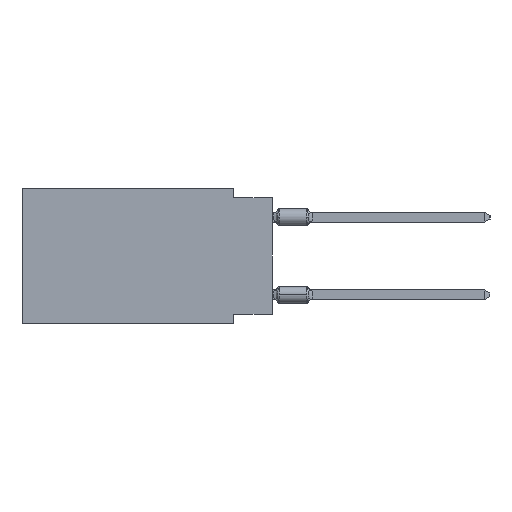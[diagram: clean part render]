
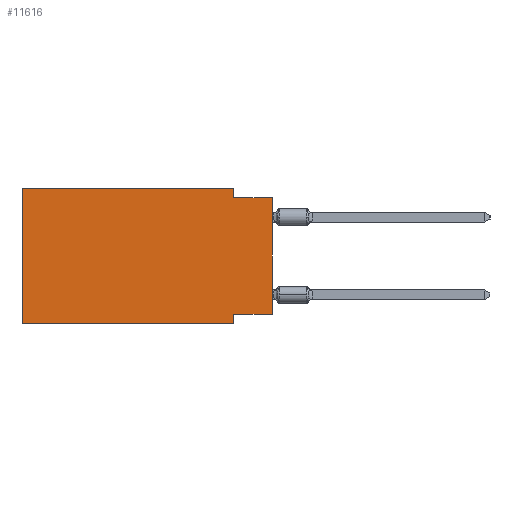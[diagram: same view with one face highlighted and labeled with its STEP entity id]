
A CAD part, left-side view. The second image highlights one B-rep face of the part: STEP entity #11616.
In plain terms, the highlighted planar face has unit normal (-1, 0, 0).
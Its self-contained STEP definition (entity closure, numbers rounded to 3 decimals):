
#1802 = CARTESIAN_POINT ( 'NONE',  ( 0., 0., 0. ) ) ;
#1859 = DIRECTION ( 'NONE',  ( 0., -1., 0. ) ) ;
#2640 = VERTEX_POINT ( 'NONE', #13204 ) ;
#3303 = ORIENTED_EDGE ( 'NONE', *, *, #38712, .F. ) ;
#4623 = VECTOR ( 'NONE', #34540, 1000. ) ;
#5333 = CARTESIAN_POINT ( 'NONE',  ( 0., 2.54, -8.89 ) ) ;
#6080 = VERTEX_POINT ( 'NONE', #53023 ) ;
#6887 = CARTESIAN_POINT ( 'NONE',  ( 0., 2.54, -8.89 ) ) ;
#7330 = ORIENTED_EDGE ( 'NONE', *, *, #44386, .F. ) ;
#8093 = CARTESIAN_POINT ( 'NONE',  ( 0., 0., -8.255 ) ) ;
#8202 = VERTEX_POINT ( 'NONE', #47140 ) ;
#8229 = DIRECTION ( 'NONE',  ( 0., 0., 1. ) ) ;
#8268 = AXIS2_PLACEMENT_3D ( 'NONE', #31419, #26337, #47799 ) ;
#9385 = ORIENTED_EDGE ( 'NONE', *, *, #18996, .F. ) ;
#10933 = LINE ( 'NONE', #6887, #17510 ) ;
#11071 = DIRECTION ( 'NONE',  ( 0., 0., -1. ) ) ;
#11616 = ADVANCED_FACE ( 'NONE', ( #34923 ), #15035, .F. ) ;
#11798 = VECTOR ( 'NONE', #13911, 1000. ) ;
#13204 = CARTESIAN_POINT ( 'NONE',  ( 0., 16.383, 0. ) ) ;
#13313 = ORIENTED_EDGE ( 'NONE', *, *, #51616, .F. ) ;
#13911 = DIRECTION ( 'NONE',  ( 0., 0., 1. ) ) ;
#15035 = PLANE ( 'NONE',  #8268 ) ;
#15107 = CARTESIAN_POINT ( 'NONE',  ( 0., 2.54, 0. ) ) ;
#15193 = EDGE_CURVE ( 'NONE', #25334, #30535, #20195, .T. ) ;
#17510 = VECTOR ( 'NONE', #26782, 1000. ) ;
#17989 = EDGE_CURVE ( 'NONE', #25334, #47056, #26521, .T. ) ;
#18152 = VECTOR ( 'NONE', #19212, 1000. ) ;
#18179 = VECTOR ( 'NONE', #8229, 1000. ) ;
#18996 = EDGE_CURVE ( 'NONE', #8202, #6080, #44637, .T. ) ;
#19212 = DIRECTION ( 'NONE',  ( 0., -1., 0. ) ) ;
#20105 = EDGE_CURVE ( 'NONE', #30535, #42771, #10933, .T. ) ;
#20195 = LINE ( 'NONE', #8093, #30067 ) ;
#21943 = VECTOR ( 'NONE', #1859, 1000. ) ;
#23225 = LINE ( 'NONE', #39637, #18152 ) ;
#25334 = VERTEX_POINT ( 'NONE', #34840 ) ;
#26337 = DIRECTION ( 'NONE',  ( 1., 0., 0. ) ) ;
#26521 = LINE ( 'NONE', #1802, #11798 ) ;
#26666 = EDGE_CURVE ( 'NONE', #28865, #42771, #46736, .T. ) ;
#26735 = LINE ( 'NONE', #46893, #4623 ) ;
#26782 = DIRECTION ( 'NONE',  ( 0., 0., -1. ) ) ;
#28865 = VERTEX_POINT ( 'NONE', #46073 ) ;
#29840 = ORIENTED_EDGE ( 'NONE', *, *, #17989, .T. ) ;
#30067 = VECTOR ( 'NONE', #49177, 1000. ) ;
#30347 = CARTESIAN_POINT ( 'NONE',  ( 0., 16.383, -8.89 ) ) ;
#30535 = VERTEX_POINT ( 'NONE', #42897 ) ;
#30917 = ORIENTED_EDGE ( 'NONE', *, *, #20105, .F. ) ;
#31419 = CARTESIAN_POINT ( 'NONE',  ( 0., 16.383, 0. ) ) ;
#34540 = DIRECTION ( 'NONE',  ( 0., -1., 0. ) ) ;
#34762 = ORIENTED_EDGE ( 'NONE', *, *, #26666, .T. ) ;
#34840 = CARTESIAN_POINT ( 'NONE',  ( 0., 0., -8.255 ) ) ;
#34923 = FACE_OUTER_BOUND ( 'NONE', #37541, .T. ) ;
#37541 = EDGE_LOOP ( 'NONE', ( #29840, #3303, #9385, #7330, #13313, #34762, #30917, #50275 ) ) ;
#38712 = EDGE_CURVE ( 'NONE', #6080, #47056, #26735, .T. ) ;
#39637 = CARTESIAN_POINT ( 'NONE',  ( 0., 16.383, 0. ) ) ;
#42771 = VERTEX_POINT ( 'NONE', #5333 ) ;
#42897 = CARTESIAN_POINT ( 'NONE',  ( 0., 2.54, -8.255 ) ) ;
#43616 = VECTOR ( 'NONE', #11071, 1000. ) ;
#44386 = EDGE_CURVE ( 'NONE', #2640, #8202, #23225, .T. ) ;
#44637 = LINE ( 'NONE', #15107, #43616 ) ;
#45025 = CARTESIAN_POINT ( 'NONE',  ( 0., 16.383, 0. ) ) ;
#46073 = CARTESIAN_POINT ( 'NONE',  ( 0., 16.383, -8.89 ) ) ;
#46736 = LINE ( 'NONE', #30347, #21943 ) ;
#46808 = CARTESIAN_POINT ( 'NONE',  ( 0., 0., -0.635 ) ) ;
#46893 = CARTESIAN_POINT ( 'NONE',  ( 0., 0., -0.635 ) ) ;
#47056 = VERTEX_POINT ( 'NONE', #46808 ) ;
#47140 = CARTESIAN_POINT ( 'NONE',  ( 0., 2.54, 0. ) ) ;
#47799 = DIRECTION ( 'NONE',  ( 0., 0., -1. ) ) ;
#49177 = DIRECTION ( 'NONE',  ( 0., 1., 0. ) ) ;
#50275 = ORIENTED_EDGE ( 'NONE', *, *, #15193, .F. ) ;
#51616 = EDGE_CURVE ( 'NONE', #28865, #2640, #53076, .T. ) ;
#53023 = CARTESIAN_POINT ( 'NONE',  ( 0., 2.54, -0.635 ) ) ;
#53076 = LINE ( 'NONE', #45025, #18179 ) ;
